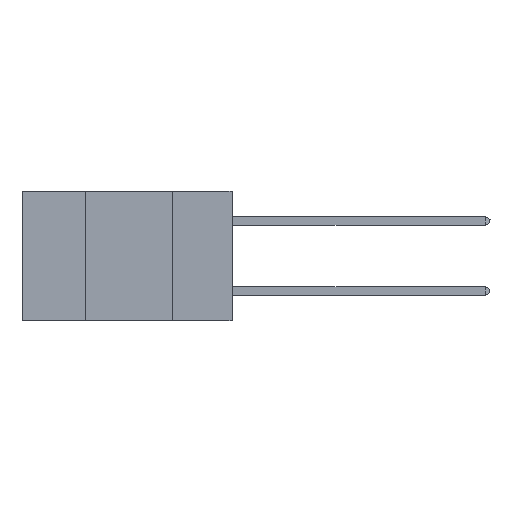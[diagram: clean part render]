
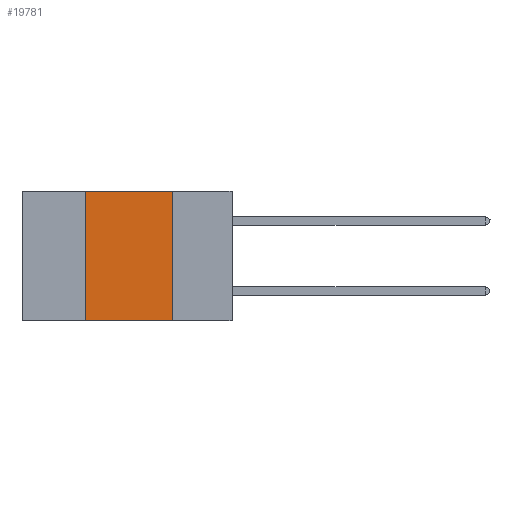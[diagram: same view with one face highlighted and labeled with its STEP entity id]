
A CAD part, left-side view. The second image highlights one B-rep face of the part: STEP entity #19781.
In plain terms, the highlighted planar face has unit normal (-1, 0, 0).
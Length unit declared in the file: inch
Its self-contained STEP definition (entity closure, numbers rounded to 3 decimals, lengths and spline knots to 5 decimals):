
#138 = CARTESIAN_POINT ( 'NONE',  ( 0., 0.17, 0. ) ) ;
#999 = EDGE_CURVE ( 'NONE', #2445, #4781, #19153, .T. ) ;
#1476 = FACE_OUTER_BOUND ( 'NONE', #15656, .T. ) ;
#1732 = VECTOR ( 'NONE', #3578, 39.37008 ) ;
#1859 = ORIENTED_EDGE ( 'NONE', *, *, #18272, .F. ) ;
#2445 = VERTEX_POINT ( 'NONE', #2895 ) ;
#2555 = VECTOR ( 'NONE', #11193, 39.37008 ) ;
#2749 = ORIENTED_EDGE ( 'NONE', *, *, #999, .T. ) ;
#2853 = PLANE ( 'NONE',  #13876 ) ;
#2895 = CARTESIAN_POINT ( 'NONE',  ( 0., 0.42, -0.37 ) ) ;
#3171 = CARTESIAN_POINT ( 'NONE',  ( 0., 0.6, 0. ) ) ;
#3567 = CARTESIAN_POINT ( 'NONE',  ( 0., 0.42, 0. ) ) ;
#3578 = DIRECTION ( 'NONE',  ( 0., -1., 0. ) ) ;
#4781 = VERTEX_POINT ( 'NONE', #18970 ) ;
#7248 = VERTEX_POINT ( 'NONE', #138 ) ;
#7695 = LINE ( 'NONE', #19893, #16876 ) ;
#8085 = ORIENTED_EDGE ( 'NONE', *, *, #15964, .F. ) ;
#8312 = CARTESIAN_POINT ( 'NONE',  ( 0., 0.6, -0.37 ) ) ;
#8624 = CARTESIAN_POINT ( 'NONE',  ( 0., 0.42, 0. ) ) ;
#8875 = CARTESIAN_POINT ( 'NONE',  ( 0., 0.6, 0. ) ) ;
#9580 = VECTOR ( 'NONE', #17119, 39.37008 ) ;
#11193 = DIRECTION ( 'NONE',  ( 0., -1., 0. ) ) ;
#13005 = DIRECTION ( 'NONE',  ( 0., 0., -1. ) ) ;
#13440 = EDGE_CURVE ( 'NONE', #2445, #16423, #18710, .T. ) ;
#13548 = DIRECTION ( 'NONE',  ( 0., 0., -1. ) ) ;
#13876 = AXIS2_PLACEMENT_3D ( 'NONE', #3171, #20442, #13548 ) ;
#15656 = EDGE_LOOP ( 'NONE', ( #1859, #8085, #17484, #2749 ) ) ;
#15964 = EDGE_CURVE ( 'NONE', #16423, #7248, #17355, .T. ) ;
#16423 = VERTEX_POINT ( 'NONE', #8624 ) ;
#16876 = VECTOR ( 'NONE', #13005, 39.37008 ) ;
#17119 = DIRECTION ( 'NONE',  ( 0., 0., 1. ) ) ;
#17355 = LINE ( 'NONE', #8875, #1732 ) ;
#17484 = ORIENTED_EDGE ( 'NONE', *, *, #13440, .F. ) ;
#18272 = EDGE_CURVE ( 'NONE', #7248, #4781, #7695, .T. ) ;
#18710 = LINE ( 'NONE', #3567, #9580 ) ;
#18970 = CARTESIAN_POINT ( 'NONE',  ( 0., 0.17, -0.37 ) ) ;
#19153 = LINE ( 'NONE', #8312, #2555 ) ;
#19781 = ADVANCED_FACE ( 'NONE', ( #1476 ), #2853, .F. ) ;
#19893 = CARTESIAN_POINT ( 'NONE',  ( 0., 0.17, 0. ) ) ;
#20442 = DIRECTION ( 'NONE',  ( 1., 0., 0. ) ) ;
